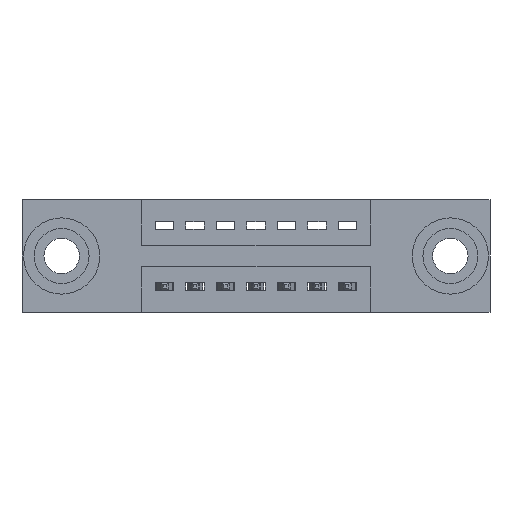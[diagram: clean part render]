
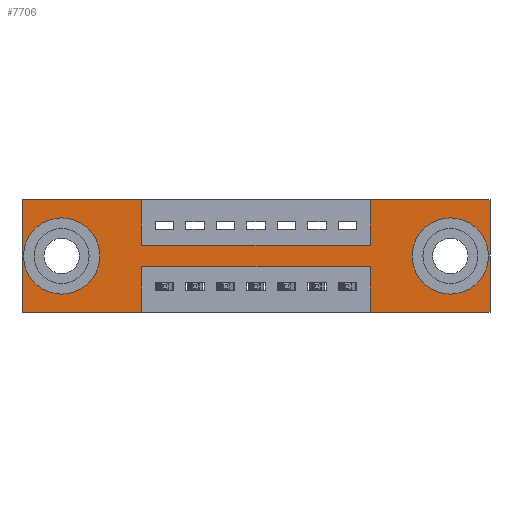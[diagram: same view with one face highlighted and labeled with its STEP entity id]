
A CAD part, front view. The second image highlights one B-rep face of the part: STEP entity #7706.
In plain terms, the highlighted planar face has unit normal (0, -1, 0).
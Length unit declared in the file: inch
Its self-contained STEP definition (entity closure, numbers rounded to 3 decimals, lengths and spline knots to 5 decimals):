
#1 = ORIENTED_EDGE ( 'NONE', *, *, #10406, .F. ) ;
#36 = VERTEX_POINT ( 'NONE', #788 ) ;
#133 = CARTESIAN_POINT ( 'NONE',  ( 0., 0., -0.37 ) ) ;
#202 = CARTESIAN_POINT ( 'NONE',  ( 0., 0., -0.37 ) ) ;
#309 = CARTESIAN_POINT ( 'NONE',  ( 1.535, 0., -0.37 ) ) ;
#348 = EDGE_CURVE ( 'NONE', #3399, #3834, #3149, .T. ) ;
#579 = VERTEX_POINT ( 'NONE', #8854 ) ;
#588 = EDGE_CURVE ( 'NONE', #3834, #1782, #9391, .T. ) ;
#743 = CARTESIAN_POINT ( 'NONE',  ( 1.405, 0., -0.185 ) ) ;
#788 = CARTESIAN_POINT ( 'NONE',  ( 0.13, 0., -0.107 ) ) ;
#854 = LINE ( 'NONE', #9653, #6507 ) ;
#865 = EDGE_LOOP ( 'NONE', ( #4296, #6516 ) ) ;
#1028 = DIRECTION ( 'NONE',  ( 0., 1., 0. ) ) ;
#1104 = EDGE_CURVE ( 'NONE', #3453, #3399, #5219, .T. ) ;
#1296 = EDGE_LOOP ( 'NONE', ( #5570, #7284, #7831, #1, #8775, #8032, #9092, #10659, #9593, #4290, #7895, #6197 ) ) ;
#1354 = VERTEX_POINT ( 'NONE', #2499 ) ;
#1586 = LINE ( 'NONE', #5459, #6485 ) ;
#1622 = DIRECTION ( 'NONE',  ( 0., 1., 0. ) ) ;
#1782 = VERTEX_POINT ( 'NONE', #8718 ) ;
#2100 = DIRECTION ( 'NONE',  ( 0., 1., 0. ) ) ;
#2242 = CARTESIAN_POINT ( 'NONE',  ( 1.535, 0., 0. ) ) ;
#2274 = DIRECTION ( 'NONE',  ( 0., 0., 1. ) ) ;
#2470 = VERTEX_POINT ( 'NONE', #8522 ) ;
#2489 = DIRECTION ( 'NONE',  ( 0., -1., 0. ) ) ;
#2499 = CARTESIAN_POINT ( 'NONE',  ( 0.13, 0., -0.263 ) ) ;
#2570 = CARTESIAN_POINT ( 'NONE',  ( 1.405, 0., -0.263 ) ) ;
#2599 = CARTESIAN_POINT ( 'NONE',  ( 0.13, 0., -0.185 ) ) ;
#2731 = LINE ( 'NONE', #7174, #10125 ) ;
#2736 = EDGE_CURVE ( 'NONE', #9506, #5507, #854, .T. ) ;
#2752 = ORIENTED_EDGE ( 'NONE', *, *, #4545, .T. ) ;
#2776 = VECTOR ( 'NONE', #5676, 39.37008 ) ;
#2877 = DIRECTION ( 'NONE',  ( -1., 0., 0. ) ) ;
#2897 = DIRECTION ( 'NONE',  ( 0., 0., -1. ) ) ;
#2941 = AXIS2_PLACEMENT_3D ( 'NONE', #133, #2489, #9182 ) ;
#2952 = LINE ( 'NONE', #202, #4900 ) ;
#2953 = EDGE_CURVE ( 'NONE', #9074, #9003, #3634, .T. ) ;
#2996 = DIRECTION ( 'NONE',  ( 0., 0., -1. ) ) ;
#3149 = LINE ( 'NONE', #7805, #8499 ) ;
#3266 = CARTESIAN_POINT ( 'NONE',  ( 0.3925, 0., -0.37 ) ) ;
#3351 = PLANE ( 'NONE',  #2941 ) ;
#3389 = DIRECTION ( 'NONE',  ( 0., 0., 1. ) ) ;
#3399 = VERTEX_POINT ( 'NONE', #8369 ) ;
#3453 = VERTEX_POINT ( 'NONE', #3469 ) ;
#3469 = CARTESIAN_POINT ( 'NONE',  ( 1.1425, 0., -0.37 ) ) ;
#3546 = CARTESIAN_POINT ( 'NONE',  ( 0., 0., 0. ) ) ;
#3634 = CIRCLE ( 'NONE', #5510, 0.078 ) ;
#3777 = CIRCLE ( 'NONE', #6529, 0.078 ) ;
#3834 = VERTEX_POINT ( 'NONE', #4918 ) ;
#4018 = AXIS2_PLACEMENT_3D ( 'NONE', #743, #1622, #2897 ) ;
#4128 = VECTOR ( 'NONE', #2996, 39.37008 ) ;
#4188 = CARTESIAN_POINT ( 'NONE',  ( 0.13, 0., -0.185 ) ) ;
#4222 = EDGE_CURVE ( 'NONE', #5507, #4888, #7794, .T. ) ;
#4290 = ORIENTED_EDGE ( 'NONE', *, *, #2736, .F. ) ;
#4296 = ORIENTED_EDGE ( 'NONE', *, *, #2953, .T. ) ;
#4442 = VECTOR ( 'NONE', #6330, 39.37008 ) ;
#4491 = EDGE_CURVE ( 'NONE', #8542, #2470, #8706, .T. ) ;
#4545 = EDGE_CURVE ( 'NONE', #36, #1354, #10640, .T. ) ;
#4633 = EDGE_CURVE ( 'NONE', #1782, #7076, #2952, .T. ) ;
#4638 = VECTOR ( 'NONE', #6571, 39.37008 ) ;
#4888 = VERTEX_POINT ( 'NONE', #8062 ) ;
#4900 = VECTOR ( 'NONE', #9217, 39.37008 ) ;
#4918 = CARTESIAN_POINT ( 'NONE',  ( 0.3925, 0., -0.22 ) ) ;
#5219 = LINE ( 'NONE', #8766, #4442 ) ;
#5227 = DIRECTION ( 'NONE',  ( 0., 1., 0. ) ) ;
#5459 = CARTESIAN_POINT ( 'NONE',  ( 0., 0., -0.37 ) ) ;
#5507 = VERTEX_POINT ( 'NONE', #8629 ) ;
#5510 = AXIS2_PLACEMENT_3D ( 'NONE', #8611, #5227, #6901 ) ;
#5570 = ORIENTED_EDGE ( 'NONE', *, *, #588, .F. ) ;
#5637 = CARTESIAN_POINT ( 'NONE',  ( 1.405, 0., -0.107 ) ) ;
#5676 = DIRECTION ( 'NONE',  ( 0., 0., -1. ) ) ;
#5905 = VECTOR ( 'NONE', #9633, 39.37008 ) ;
#5979 = VERTEX_POINT ( 'NONE', #309 ) ;
#6161 = LINE ( 'NONE', #8246, #8510 ) ;
#6191 = DIRECTION ( 'NONE',  ( 0., 0., 1. ) ) ;
#6193 = CARTESIAN_POINT ( 'NONE',  ( 1.1425, 0., 0. ) ) ;
#6197 = ORIENTED_EDGE ( 'NONE', *, *, #4633, .F. ) ;
#6330 = DIRECTION ( 'NONE',  ( 0., 0., 1. ) ) ;
#6485 = VECTOR ( 'NONE', #9990, 39.37008 ) ;
#6507 = VECTOR ( 'NONE', #9766, 39.37008 ) ;
#6516 = ORIENTED_EDGE ( 'NONE', *, *, #9926, .T. ) ;
#6529 = AXIS2_PLACEMENT_3D ( 'NONE', #4188, #2100, #8783 ) ;
#6571 = DIRECTION ( 'NONE',  ( 1., 0., 0. ) ) ;
#6901 = DIRECTION ( 'NONE',  ( 0., 0., -1. ) ) ;
#6934 = EDGE_CURVE ( 'NONE', #7076, #9506, #9833, .T. ) ;
#7076 = VERTEX_POINT ( 'NONE', #9609 ) ;
#7100 = ORIENTED_EDGE ( 'NONE', *, *, #9258, .T. ) ;
#7174 = CARTESIAN_POINT ( 'NONE',  ( 1.1425, 0., 0. ) ) ;
#7284 = ORIENTED_EDGE ( 'NONE', *, *, #348, .F. ) ;
#7465 = FACE_OUTER_BOUND ( 'NONE', #1296, .T. ) ;
#7480 = EDGE_CURVE ( 'NONE', #2470, #5979, #8133, .T. ) ;
#7519 = CARTESIAN_POINT ( 'NONE',  ( 0., 0., 0. ) ) ;
#7693 = EDGE_CURVE ( 'NONE', #4888, #579, #6161, .T. ) ;
#7706 = ADVANCED_FACE ( 'NONE', ( #7991, #9683, #7465 ), #3351, .T. ) ;
#7794 = LINE ( 'NONE', #8002, #4128 ) ;
#7805 = CARTESIAN_POINT ( 'NONE',  ( 0.3925, 0., -0.22 ) ) ;
#7831 = ORIENTED_EDGE ( 'NONE', *, *, #1104, .F. ) ;
#7895 = ORIENTED_EDGE ( 'NONE', *, *, #6934, .F. ) ;
#7991 = FACE_BOUND ( 'NONE', #865, .T. ) ;
#8002 = CARTESIAN_POINT ( 'NONE',  ( 0.3925, 0., 0. ) ) ;
#8032 = ORIENTED_EDGE ( 'NONE', *, *, #4491, .F. ) ;
#8062 = CARTESIAN_POINT ( 'NONE',  ( 0.3925, 0., -0.15 ) ) ;
#8133 = LINE ( 'NONE', #2242, #5905 ) ;
#8246 = CARTESIAN_POINT ( 'NONE',  ( 0.3925, 0., -0.15 ) ) ;
#8369 = CARTESIAN_POINT ( 'NONE',  ( 1.1425, 0., -0.22 ) ) ;
#8499 = VECTOR ( 'NONE', #2877, 39.37008 ) ;
#8510 = VECTOR ( 'NONE', #9084, 39.37008 ) ;
#8522 = CARTESIAN_POINT ( 'NONE',  ( 1.535, 0., 0. ) ) ;
#8542 = VERTEX_POINT ( 'NONE', #6193 ) ;
#8611 = CARTESIAN_POINT ( 'NONE',  ( 1.405, 0., -0.185 ) ) ;
#8629 = CARTESIAN_POINT ( 'NONE',  ( 0.3925, 0., 0. ) ) ;
#8650 = VECTOR ( 'NONE', #6191, 39.37008 ) ;
#8706 = LINE ( 'NONE', #7519, #4638 ) ;
#8718 = CARTESIAN_POINT ( 'NONE',  ( 0.3925, 0., -0.37 ) ) ;
#8766 = CARTESIAN_POINT ( 'NONE',  ( 1.1425, 0., -0.37 ) ) ;
#8775 = ORIENTED_EDGE ( 'NONE', *, *, #7480, .F. ) ;
#8783 = DIRECTION ( 'NONE',  ( 0., 0., 1. ) ) ;
#8854 = CARTESIAN_POINT ( 'NONE',  ( 1.1425, 0., -0.15 ) ) ;
#9003 = VERTEX_POINT ( 'NONE', #2570 ) ;
#9074 = VERTEX_POINT ( 'NONE', #5637 ) ;
#9084 = DIRECTION ( 'NONE',  ( 1., 0., 0. ) ) ;
#9092 = ORIENTED_EDGE ( 'NONE', *, *, #10070, .F. ) ;
#9182 = DIRECTION ( 'NONE',  ( 0., 0., -1. ) ) ;
#9217 = DIRECTION ( 'NONE',  ( -1., 0., 0. ) ) ;
#9258 = EDGE_CURVE ( 'NONE', #1354, #36, #3777, .T. ) ;
#9344 = CIRCLE ( 'NONE', #4018, 0.078 ) ;
#9391 = LINE ( 'NONE', #3266, #2776 ) ;
#9506 = VERTEX_POINT ( 'NONE', #9845 ) ;
#9593 = ORIENTED_EDGE ( 'NONE', *, *, #4222, .F. ) ;
#9609 = CARTESIAN_POINT ( 'NONE',  ( 0., 0., -0.37 ) ) ;
#9633 = DIRECTION ( 'NONE',  ( 0., 0., -1. ) ) ;
#9653 = CARTESIAN_POINT ( 'NONE',  ( 0., 0., 0. ) ) ;
#9683 = FACE_BOUND ( 'NONE', #9948, .T. ) ;
#9766 = DIRECTION ( 'NONE',  ( 1., 0., 0. ) ) ;
#9833 = LINE ( 'NONE', #3546, #8650 ) ;
#9845 = CARTESIAN_POINT ( 'NONE',  ( 0., 0., 0. ) ) ;
#9921 = AXIS2_PLACEMENT_3D ( 'NONE', #2599, #1028, #3389 ) ;
#9926 = EDGE_CURVE ( 'NONE', #9003, #9074, #9344, .T. ) ;
#9948 = EDGE_LOOP ( 'NONE', ( #2752, #7100 ) ) ;
#9990 = DIRECTION ( 'NONE',  ( -1., 0., 0. ) ) ;
#10070 = EDGE_CURVE ( 'NONE', #579, #8542, #2731, .T. ) ;
#10125 = VECTOR ( 'NONE', #2274, 39.37008 ) ;
#10406 = EDGE_CURVE ( 'NONE', #5979, #3453, #1586, .T. ) ;
#10640 = CIRCLE ( 'NONE', #9921, 0.078 ) ;
#10659 = ORIENTED_EDGE ( 'NONE', *, *, #7693, .F. ) ;
